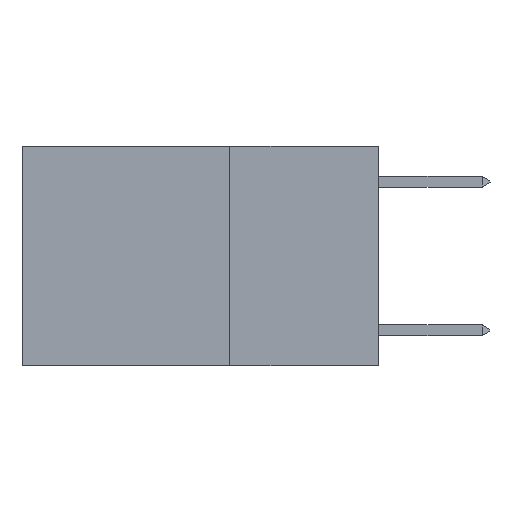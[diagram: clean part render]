
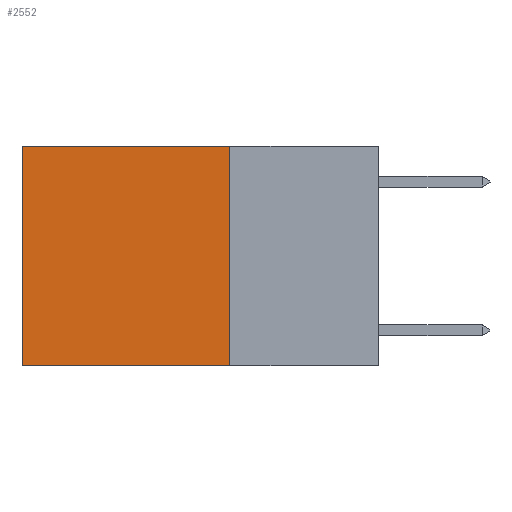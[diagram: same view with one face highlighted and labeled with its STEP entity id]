
A CAD part, left-side view. The second image highlights one B-rep face of the part: STEP entity #2552.
In plain terms, the highlighted planar face has unit normal (-1, 0, 0).
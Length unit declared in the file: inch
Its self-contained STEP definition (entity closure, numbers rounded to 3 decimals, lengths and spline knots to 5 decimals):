
#30 = EDGE_CURVE ( 'NONE', #6102, #85, #4968, .T. ) ;
#85 = VERTEX_POINT ( 'NONE', #9854 ) ;
#668 = FACE_OUTER_BOUND ( 'NONE', #9760, .T. ) ;
#1130 = CARTESIAN_POINT ( 'NONE',  ( 0.2625, 0.25, 0. ) ) ;
#1247 = CARTESIAN_POINT ( 'NONE',  ( 0.2625, 0.25, -0.37 ) ) ;
#1639 = DIRECTION ( 'NONE',  ( 0., 0., -1. ) ) ;
#2552 = ADVANCED_FACE ( 'NONE', ( #668 ), #8403, .F. ) ;
#3039 = VECTOR ( 'NONE', #5514, 39.37008 ) ;
#3296 = LINE ( 'NONE', #3881, #3039 ) ;
#3301 = ORIENTED_EDGE ( 'NONE', *, *, #7361, .T. ) ;
#3320 = CARTESIAN_POINT ( 'NONE',  ( 0.2625, 0.25, 0. ) ) ;
#3548 = ORIENTED_EDGE ( 'NONE', *, *, #7694, .T. ) ;
#3881 = CARTESIAN_POINT ( 'NONE',  ( 0.2625, 0.6, 0. ) ) ;
#4053 = VECTOR ( 'NONE', #6879, 39.37008 ) ;
#4461 = CARTESIAN_POINT ( 'NONE',  ( 0.2625, 0.25, -0.37 ) ) ;
#4873 = DIRECTION ( 'NONE',  ( 1., 0., 0. ) ) ;
#4912 = DIRECTION ( 'NONE',  ( 0., 1., 0. ) ) ;
#4968 = LINE ( 'NONE', #1247, #8713 ) ;
#4987 = VECTOR ( 'NONE', #7381, 39.37008 ) ;
#5351 = ORIENTED_EDGE ( 'NONE', *, *, #30, .F. ) ;
#5514 = DIRECTION ( 'NONE',  ( 0., 0., -1. ) ) ;
#6028 = LINE ( 'NONE', #8355, #4053 ) ;
#6102 = VERTEX_POINT ( 'NONE', #4461 ) ;
#6879 = DIRECTION ( 'NONE',  ( 0., 0., -1. ) ) ;
#7173 = CARTESIAN_POINT ( 'NONE',  ( 0.2625, 0.6, 0. ) ) ;
#7230 = EDGE_CURVE ( 'NONE', #8876, #6102, #6028, .T. ) ;
#7361 = EDGE_CURVE ( 'NONE', #9443, #85, #3296, .T. ) ;
#7381 = DIRECTION ( 'NONE',  ( 0., 1., 0. ) ) ;
#7694 = EDGE_CURVE ( 'NONE', #8876, #9443, #8969, .T. ) ;
#8171 = AXIS2_PLACEMENT_3D ( 'NONE', #3320, #4873, #1639 ) ;
#8355 = CARTESIAN_POINT ( 'NONE',  ( 0.2625, 0.25, 0. ) ) ;
#8403 = PLANE ( 'NONE',  #8171 ) ;
#8591 = CARTESIAN_POINT ( 'NONE',  ( 0.2625, 0.25, 0. ) ) ;
#8713 = VECTOR ( 'NONE', #4912, 39.37008 ) ;
#8876 = VERTEX_POINT ( 'NONE', #8591 ) ;
#8969 = LINE ( 'NONE', #1130, #4987 ) ;
#9324 = ORIENTED_EDGE ( 'NONE', *, *, #7230, .F. ) ;
#9443 = VERTEX_POINT ( 'NONE', #7173 ) ;
#9760 = EDGE_LOOP ( 'NONE', ( #3301, #5351, #9324, #3548 ) ) ;
#9854 = CARTESIAN_POINT ( 'NONE',  ( 0.2625, 0.6, -0.37 ) ) ;
